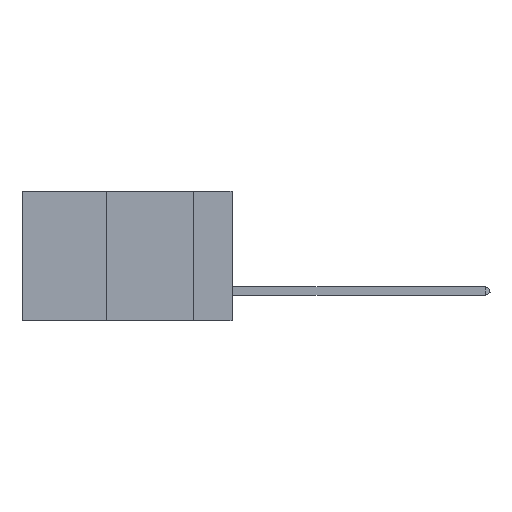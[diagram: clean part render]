
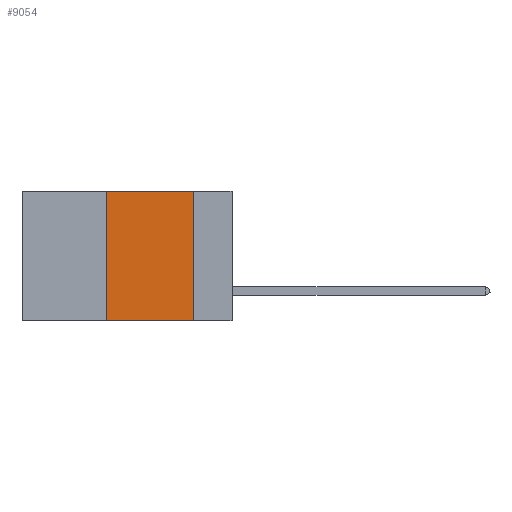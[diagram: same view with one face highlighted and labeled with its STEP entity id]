
A CAD part, left-side view. The second image highlights one B-rep face of the part: STEP entity #9054.
In plain terms, the highlighted planar face has unit normal (-1, 0, 0).
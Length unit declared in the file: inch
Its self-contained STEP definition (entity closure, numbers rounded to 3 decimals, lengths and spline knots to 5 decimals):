
#76 = VERTEX_POINT ( 'NONE', #4590 ) ;
#706 = CARTESIAN_POINT ( 'NONE',  ( 0., 0.11, -0.37 ) ) ;
#1152 = LINE ( 'NONE', #1468, #1893 ) ;
#1468 = CARTESIAN_POINT ( 'NONE',  ( 0., 0.36, 0. ) ) ;
#1893 = VECTOR ( 'NONE', #2379, 39.37008 ) ;
#2185 = DIRECTION ( 'NONE',  ( 0., 0., -1. ) ) ;
#2379 = DIRECTION ( 'NONE',  ( 0., 0., 1. ) ) ;
#2480 = EDGE_CURVE ( 'NONE', #3584, #4238, #1152, .T. ) ;
#2635 = ORIENTED_EDGE ( 'NONE', *, *, #3700, .F. ) ;
#2998 = VECTOR ( 'NONE', #10244, 39.37008 ) ;
#3088 = VECTOR ( 'NONE', #2185, 39.37008 ) ;
#3584 = VERTEX_POINT ( 'NONE', #8476 ) ;
#3700 = EDGE_CURVE ( 'NONE', #76, #10281, #5671, .T. ) ;
#4238 = VERTEX_POINT ( 'NONE', #10539 ) ;
#4574 = LINE ( 'NONE', #10356, #10522 ) ;
#4590 = CARTESIAN_POINT ( 'NONE',  ( 0., 0.11, 0. ) ) ;
#5322 = ORIENTED_EDGE ( 'NONE', *, *, #12410, .T. ) ;
#5671 = LINE ( 'NONE', #10020, #3088 ) ;
#6059 = DIRECTION ( 'NONE',  ( 0., 0., -1. ) ) ;
#6448 = EDGE_CURVE ( 'NONE', #4238, #76, #10933, .T. ) ;
#6489 = ORIENTED_EDGE ( 'NONE', *, *, #2480, .F. ) ;
#7160 = PLANE ( 'NONE',  #8214 ) ;
#7809 = ORIENTED_EDGE ( 'NONE', *, *, #6448, .F. ) ;
#8010 = CARTESIAN_POINT ( 'NONE',  ( 0., 0.6, 0. ) ) ;
#8214 = AXIS2_PLACEMENT_3D ( 'NONE', #8010, #11925, #6059 ) ;
#8476 = CARTESIAN_POINT ( 'NONE',  ( 0., 0.36, -0.37 ) ) ;
#9054 = ADVANCED_FACE ( 'NONE', ( #10929 ), #7160, .F. ) ;
#9235 = CARTESIAN_POINT ( 'NONE',  ( 0., 0.6, 0. ) ) ;
#10020 = CARTESIAN_POINT ( 'NONE',  ( 0., 0.11, 0. ) ) ;
#10244 = DIRECTION ( 'NONE',  ( 0., -1., 0. ) ) ;
#10281 = VERTEX_POINT ( 'NONE', #706 ) ;
#10356 = CARTESIAN_POINT ( 'NONE',  ( 0., 0.6, -0.37 ) ) ;
#10522 = VECTOR ( 'NONE', #10895, 39.37008 ) ;
#10539 = CARTESIAN_POINT ( 'NONE',  ( 0., 0.36, 0. ) ) ;
#10895 = DIRECTION ( 'NONE',  ( 0., -1., 0. ) ) ;
#10929 = FACE_OUTER_BOUND ( 'NONE', #11312, .T. ) ;
#10933 = LINE ( 'NONE', #9235, #2998 ) ;
#11312 = EDGE_LOOP ( 'NONE', ( #2635, #7809, #6489, #5322 ) ) ;
#11925 = DIRECTION ( 'NONE',  ( 1., 0., 0. ) ) ;
#12410 = EDGE_CURVE ( 'NONE', #3584, #10281, #4574, .T. ) ;
